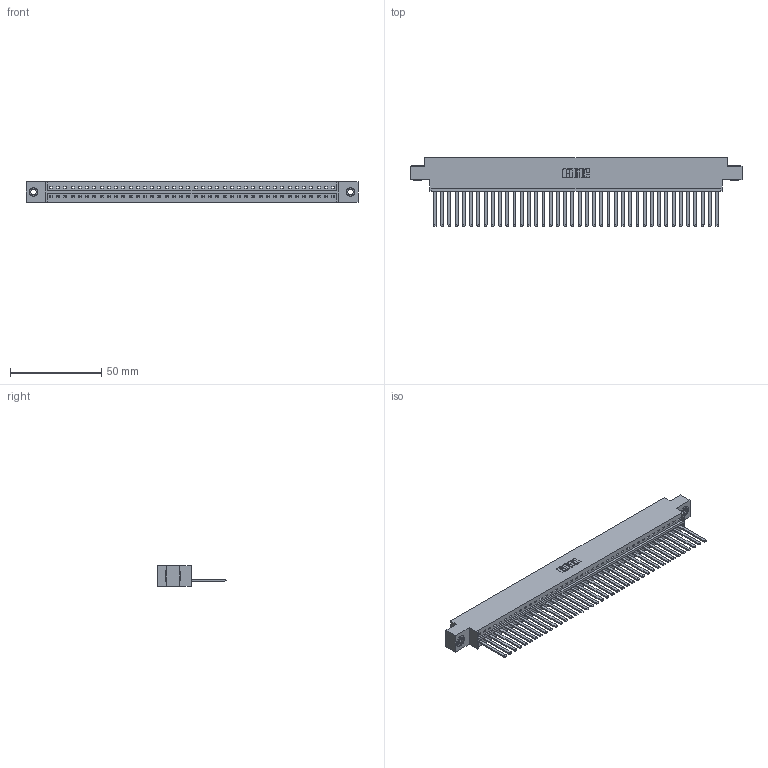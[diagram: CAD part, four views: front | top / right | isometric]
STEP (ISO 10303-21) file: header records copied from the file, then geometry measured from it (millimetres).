
FILE_DESCRIPTION (( 'STEP AP203' ), '1' );
FILE_NAME ('336-040-541-603.STEP', '2020-08-07T23:15:44', ( '' ), ( '' ), 'SwSTEP 2.0', 'SolidWorks 2020', '' );
FILE_SCHEMA (( 'CONFIG_CONTROL_DESIGN' ));
Length unit declared in the file: inch
Products named in the file (4): 336-290-001_336-290-541; 345-250-002_345-250-002-102; 336 Part_Offset - .156 Dia - TH; 336-040-541-603
Assembly tree (43 placements, depth 2):
  336-040-541-603
    336 Part_Offset - .156 Dia - TH
    336-290-001_336-290-541  x40
    345-250-002_345-250-002-102  x2
Bounding box: 181.89 x 37.34 x 11.1 mm (x, y, z)
Volume: 26462.7 mm3; surface area: 29089.8 mm2
Topology: 43 solids, 43 shells, 2156 faces, 6559 edges, 4342 vertices
Faces by surface type: plane 1444, cylinder 704, cone 8
Entity records: 30493 total; most frequent: CARTESIAN_POINT 5372, ORIENTED_EDGE 5242, DIRECTION 4463, EDGE_CURVE 2621, VECTOR 2465, LINE 2465, VERTEX_POINT 1744, AXIS2_PLACEMENT_3D 999
